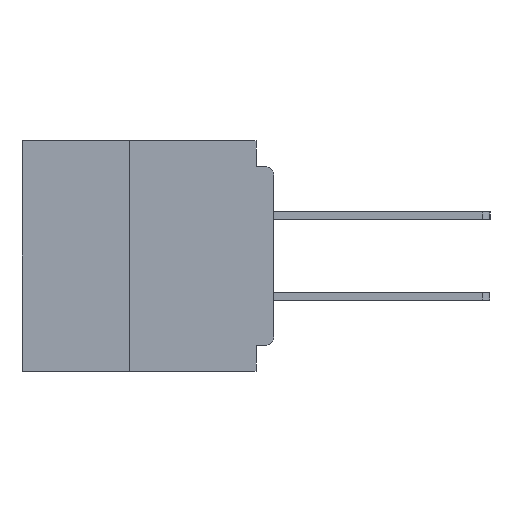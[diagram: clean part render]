
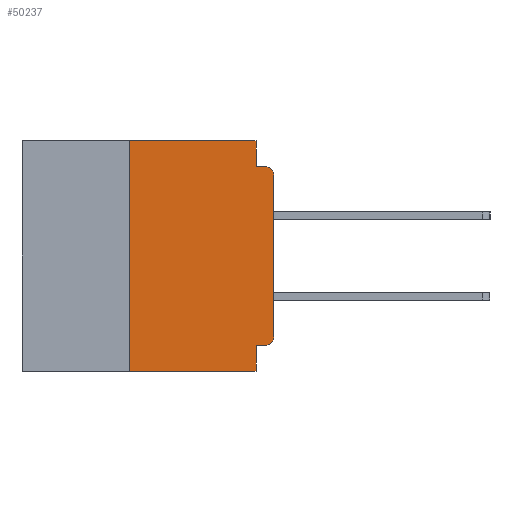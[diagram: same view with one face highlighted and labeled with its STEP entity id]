
A CAD part, left-side view. The second image highlights one B-rep face of the part: STEP entity #50237.
In plain terms, the highlighted planar face has unit normal (-1, 0, 0).
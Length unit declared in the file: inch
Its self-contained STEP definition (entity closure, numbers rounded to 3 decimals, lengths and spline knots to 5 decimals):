
#64 = LINE ( 'NONE', #21841, #39498 ) ;
#243 = CARTESIAN_POINT ( 'NONE',  ( 0., 0.437, 0. ) ) ;
#687 = VERTEX_POINT ( 'NONE', #41676 ) ;
#2134 = VECTOR ( 'NONE', #18896, 39.37008 ) ;
#3163 = DIRECTION ( 'NONE',  ( 0., 1., 0. ) ) ;
#4967 = VERTEX_POINT ( 'NONE', #8699 ) ;
#5139 = VECTOR ( 'NONE', #52321, 39.37008 ) ;
#5246 = DIRECTION ( 'NONE',  ( 0., 0., -1. ) ) ;
#7565 = ORIENTED_EDGE ( 'NONE', *, *, #48419, .T. ) ;
#7980 = CARTESIAN_POINT ( 'NONE',  ( 0., 0.437, -0.4 ) ) ;
#8049 = VECTOR ( 'NONE', #62869, 39.37008 ) ;
#8699 = CARTESIAN_POINT ( 'NONE',  ( 0., 0.031, -0.355 ) ) ;
#9403 = VERTEX_POINT ( 'NONE', #32103 ) ;
#9621 = LINE ( 'NONE', #53029, #8049 ) ;
#9819 = CARTESIAN_POINT ( 'NONE',  ( 0., 0.25, -0.4 ) ) ;
#11454 = ORIENTED_EDGE ( 'NONE', *, *, #25459, .F. ) ;
#13026 = LINE ( 'NONE', #62181, #53891 ) ;
#15031 = EDGE_CURVE ( 'NONE', #46730, #687, #18303, .T. ) ;
#15433 = AXIS2_PLACEMENT_3D ( 'NONE', #243, #34836, #5246 ) ;
#18176 = DIRECTION ( 'NONE',  ( -1., 0., 0. ) ) ;
#18250 = VERTEX_POINT ( 'NONE', #42459 ) ;
#18303 = LINE ( 'NONE', #7980, #5139 ) ;
#18896 = DIRECTION ( 'NONE',  ( 0., 0., 1. ) ) ;
#19066 = CARTESIAN_POINT ( 'NONE',  ( 0., 0.015, -0.34 ) ) ;
#19641 = VECTOR ( 'NONE', #62944, 39.37008 ) ;
#20133 = VECTOR ( 'NONE', #24867, 39.37008 ) ;
#21841 = CARTESIAN_POINT ( 'NONE',  ( 0., 0.031, -0.4 ) ) ;
#23012 = DIRECTION ( 'NONE',  ( 0., -1., 0. ) ) ;
#23471 = FACE_OUTER_BOUND ( 'NONE', #57147, .T. ) ;
#24042 = DIRECTION ( 'NONE',  ( 0., 0., -1. ) ) ;
#24867 = DIRECTION ( 'NONE',  ( 0., 0., 1. ) ) ;
#24957 = PLANE ( 'NONE',  #15433 ) ;
#25113 = VECTOR ( 'NONE', #23012, 39.37008 ) ;
#25459 = EDGE_CURVE ( 'NONE', #46701, #45881, #9621, .T. ) ;
#26412 = CARTESIAN_POINT ( 'NONE',  ( 0., 0.015, -0.045 ) ) ;
#27270 = EDGE_CURVE ( 'NONE', #32493, #9403, #34954, .T. ) ;
#27629 = EDGE_CURVE ( 'NONE', #4967, #687, #64, .T. ) ;
#28194 = AXIS2_PLACEMENT_3D ( 'NONE', #47604, #18176, #52570 ) ;
#28379 = CARTESIAN_POINT ( 'NONE',  ( 0., 0., -0.06 ) ) ;
#29275 = EDGE_CURVE ( 'NONE', #39841, #32200, #36416, .T. ) ;
#32103 = CARTESIAN_POINT ( 'NONE',  ( 0., 0., -0.34 ) ) ;
#32200 = VERTEX_POINT ( 'NONE', #26412 ) ;
#32493 = VERTEX_POINT ( 'NONE', #52989 ) ;
#34126 = ORIENTED_EDGE ( 'NONE', *, *, #29275, .T. ) ;
#34208 = CARTESIAN_POINT ( 'NONE',  ( 0., 0.031, 0. ) ) ;
#34836 = DIRECTION ( 'NONE',  ( 1., 0., 0. ) ) ;
#34954 = CIRCLE ( 'NONE', #52309, 0.015 ) ;
#36416 = CIRCLE ( 'NONE', #28194, 0.015 ) ;
#39498 = VECTOR ( 'NONE', #56213, 39.37008 ) ;
#39841 = VERTEX_POINT ( 'NONE', #28379 ) ;
#40022 = LINE ( 'NONE', #43412, #2134 ) ;
#41327 = ORIENTED_EDGE ( 'NONE', *, *, #27270, .T. ) ;
#41676 = CARTESIAN_POINT ( 'NONE',  ( 0., 0.031, -0.4 ) ) ;
#42459 = CARTESIAN_POINT ( 'NONE',  ( 0., 0.25, 0. ) ) ;
#43412 = CARTESIAN_POINT ( 'NONE',  ( 0., 0., 0. ) ) ;
#44447 = ORIENTED_EDGE ( 'NONE', *, *, #15031, .T. ) ;
#44728 = LINE ( 'NONE', #54301, #20133 ) ;
#45766 = LINE ( 'NONE', #58041, #19641 ) ;
#45881 = VERTEX_POINT ( 'NONE', #57036 ) ;
#46701 = VERTEX_POINT ( 'NONE', #34208 ) ;
#46730 = VERTEX_POINT ( 'NONE', #9819 ) ;
#47494 = CARTESIAN_POINT ( 'NONE',  ( 0., 0., -0.045 ) ) ;
#47604 = CARTESIAN_POINT ( 'NONE',  ( 0., 0.015, -0.06 ) ) ;
#47743 = ORIENTED_EDGE ( 'NONE', *, *, #63277, .F. ) ;
#48419 = EDGE_CURVE ( 'NONE', #9403, #39841, #40022, .T. ) ;
#50092 = EDGE_CURVE ( 'NONE', #18250, #46701, #45766, .T. ) ;
#50237 = ADVANCED_FACE ( 'NONE', ( #23471 ), #24957, .F. ) ;
#52200 = ORIENTED_EDGE ( 'NONE', *, *, #57267, .F. ) ;
#52309 = AXIS2_PLACEMENT_3D ( 'NONE', #19066, #53482, #24042 ) ;
#52321 = DIRECTION ( 'NONE',  ( 0., -1., 0. ) ) ;
#52570 = DIRECTION ( 'NONE',  ( 0., 0., -1. ) ) ;
#52761 = LINE ( 'NONE', #47494, #25113 ) ;
#52989 = CARTESIAN_POINT ( 'NONE',  ( 0., 0.015, -0.355 ) ) ;
#53029 = CARTESIAN_POINT ( 'NONE',  ( 0., 0.031, 0. ) ) ;
#53482 = DIRECTION ( 'NONE',  ( -1., 0., 0. ) ) ;
#53891 = VECTOR ( 'NONE', #3163, 39.37008 ) ;
#54301 = CARTESIAN_POINT ( 'NONE',  ( 0., 0.25, -0.4 ) ) ;
#54368 = ORIENTED_EDGE ( 'NONE', *, *, #56508, .F. ) ;
#56213 = DIRECTION ( 'NONE',  ( 0., 0., -1. ) ) ;
#56508 = EDGE_CURVE ( 'NONE', #46730, #18250, #44728, .T. ) ;
#57036 = CARTESIAN_POINT ( 'NONE',  ( 0., 0.031, -0.045 ) ) ;
#57147 = EDGE_LOOP ( 'NONE', ( #7565, #34126, #47743, #11454, #61475, #54368, #44447, #62716, #52200, #41327 ) ) ;
#57267 = EDGE_CURVE ( 'NONE', #32493, #4967, #13026, .T. ) ;
#58041 = CARTESIAN_POINT ( 'NONE',  ( 0., 0.437, 0. ) ) ;
#61475 = ORIENTED_EDGE ( 'NONE', *, *, #50092, .F. ) ;
#62181 = CARTESIAN_POINT ( 'NONE',  ( 0., 0., -0.355 ) ) ;
#62716 = ORIENTED_EDGE ( 'NONE', *, *, #27629, .F. ) ;
#62869 = DIRECTION ( 'NONE',  ( 0., 0., -1. ) ) ;
#62944 = DIRECTION ( 'NONE',  ( 0., -1., 0. ) ) ;
#63277 = EDGE_CURVE ( 'NONE', #45881, #32200, #52761, .T. ) ;
